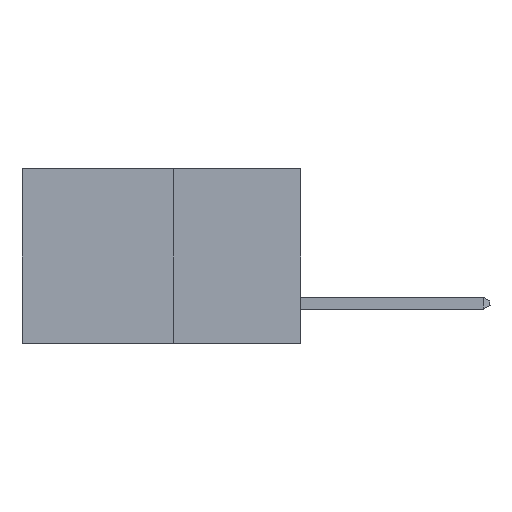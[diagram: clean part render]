
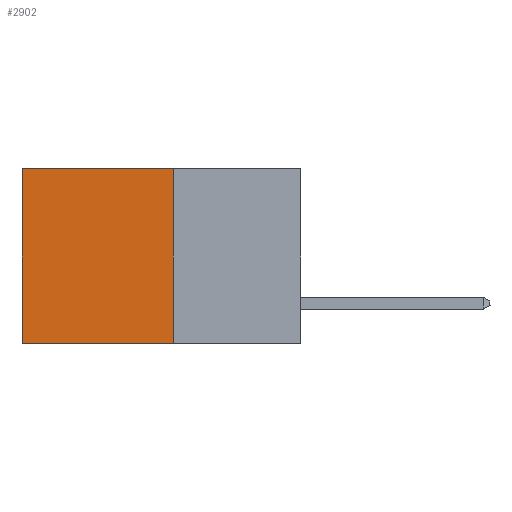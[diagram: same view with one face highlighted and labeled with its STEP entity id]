
A CAD part, left-side view. The second image highlights one B-rep face of the part: STEP entity #2902.
In plain terms, the highlighted planar face has unit normal (-1, 0, 0).
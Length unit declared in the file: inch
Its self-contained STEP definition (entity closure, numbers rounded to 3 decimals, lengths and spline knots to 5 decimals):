
#6 = LINE ( 'NONE', #20288, #14543 ) ;
#576 = CARTESIAN_POINT ( 'NONE',  ( 0.277, 0.27, -0.37 ) ) ;
#1635 = CARTESIAN_POINT ( 'NONE',  ( 0.277, 0.27, -0.37 ) ) ;
#1809 = ORIENTED_EDGE ( 'NONE', *, *, #16524, .T. ) ;
#2902 = ADVANCED_FACE ( 'NONE', ( #11987 ), #22583, .F. ) ;
#3202 = LINE ( 'NONE', #576, #23828 ) ;
#4001 = VECTOR ( 'NONE', #22040, 39.37008 ) ;
#4455 = LINE ( 'NONE', #16525, #23882 ) ;
#4578 = LINE ( 'NONE', #18298, #4001 ) ;
#4711 = EDGE_CURVE ( 'NONE', #15959, #11439, #6, .T. ) ;
#5161 = DIRECTION ( 'NONE',  ( 0., 0., -1. ) ) ;
#5626 = VERTEX_POINT ( 'NONE', #13793 ) ;
#5999 = VERTEX_POINT ( 'NONE', #23040 ) ;
#7624 = DIRECTION ( 'NONE',  ( 1., 0., 0. ) ) ;
#7941 = ORIENTED_EDGE ( 'NONE', *, *, #21550, .F. ) ;
#8122 = DIRECTION ( 'NONE',  ( 0., 0., -1. ) ) ;
#9081 = EDGE_CURVE ( 'NONE', #5626, #11439, #4455, .T. ) ;
#9888 = EDGE_LOOP ( 'NONE', ( #18252, #16059, #7941, #1809 ) ) ;
#11439 = VERTEX_POINT ( 'NONE', #17724 ) ;
#11987 = FACE_OUTER_BOUND ( 'NONE', #9888, .T. ) ;
#13793 = CARTESIAN_POINT ( 'NONE',  ( 0.277, 0.59, 0. ) ) ;
#14543 = VECTOR ( 'NONE', #22161, 39.37008 ) ;
#15959 = VERTEX_POINT ( 'NONE', #1635 ) ;
#16059 = ORIENTED_EDGE ( 'NONE', *, *, #4711, .F. ) ;
#16524 = EDGE_CURVE ( 'NONE', #5999, #5626, #4578, .T. ) ;
#16525 = CARTESIAN_POINT ( 'NONE',  ( 0.277, 0.59, -0.37 ) ) ;
#17014 = AXIS2_PLACEMENT_3D ( 'NONE', #17039, #7624, #20785 ) ;
#17039 = CARTESIAN_POINT ( 'NONE',  ( 0.277, 0.27, -0.37 ) ) ;
#17724 = CARTESIAN_POINT ( 'NONE',  ( 0.277, 0.59, -0.37 ) ) ;
#18252 = ORIENTED_EDGE ( 'NONE', *, *, #9081, .T. ) ;
#18298 = CARTESIAN_POINT ( 'NONE',  ( 0.277, 0.27, 0. ) ) ;
#20288 = CARTESIAN_POINT ( 'NONE',  ( 0.277, 0.27, -0.37 ) ) ;
#20785 = DIRECTION ( 'NONE',  ( 0., 0., -1. ) ) ;
#21550 = EDGE_CURVE ( 'NONE', #5999, #15959, #3202, .T. ) ;
#22040 = DIRECTION ( 'NONE',  ( 0., 1., 0. ) ) ;
#22161 = DIRECTION ( 'NONE',  ( 0., 1., 0. ) ) ;
#22583 = PLANE ( 'NONE',  #17014 ) ;
#23040 = CARTESIAN_POINT ( 'NONE',  ( 0.277, 0.27, 0. ) ) ;
#23828 = VECTOR ( 'NONE', #8122, 39.37008 ) ;
#23882 = VECTOR ( 'NONE', #5161, 39.37008 ) ;
